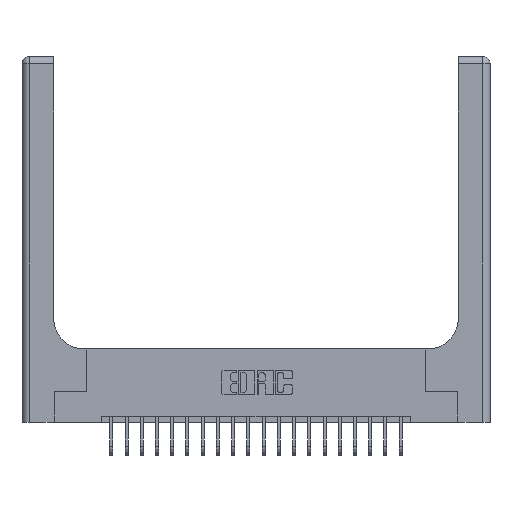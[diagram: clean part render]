
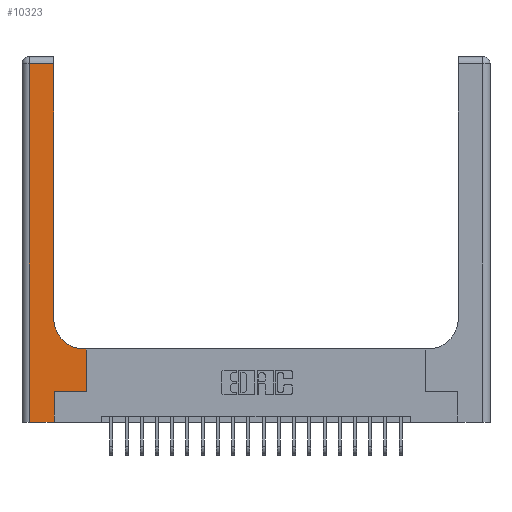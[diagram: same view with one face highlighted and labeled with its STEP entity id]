
A CAD part, top view. The second image highlights one B-rep face of the part: STEP entity #10323.
In plain terms, the highlighted planar face has unit normal (0, 0, 1).
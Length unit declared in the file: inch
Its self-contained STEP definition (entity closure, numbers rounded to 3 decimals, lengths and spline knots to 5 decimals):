
#40 = LINE ( 'NONE', #17816, #15562 ) ;
#163 = CARTESIAN_POINT ( 'NONE',  ( 0., 0., 0.37 ) ) ;
#220 = LINE ( 'NONE', #3405, #14856 ) ;
#269 = DIRECTION ( 'NONE',  ( 1., 0., 0. ) ) ;
#951 = VECTOR ( 'NONE', #11304, 39.37008 ) ;
#1153 = VECTOR ( 'NONE', #1521, 39.37008 ) ;
#1199 = FACE_OUTER_BOUND ( 'NONE', #8722, .T. ) ;
#1295 = EDGE_CURVE ( 'NONE', #9481, #20837, #11228, .T. ) ;
#1521 = DIRECTION ( 'NONE',  ( 0., 1., 0. ) ) ;
#1726 = VECTOR ( 'NONE', #14231, 39.37008 ) ;
#2073 = ORIENTED_EDGE ( 'NONE', *, *, #12295, .T. ) ;
#2400 = VECTOR ( 'NONE', #5917, 39.37008 ) ;
#2632 = CARTESIAN_POINT ( 'NONE',  ( 0.528, 0.6, 0.37 ) ) ;
#2777 = CARTESIAN_POINT ( 'NONE',  ( 0.265, 0.25, 0.37 ) ) ;
#2857 = EDGE_CURVE ( 'NONE', #16329, #14969, #40, .T. ) ;
#2881 = EDGE_CURVE ( 'NONE', #20624, #17365, #4722, .T. ) ;
#3127 = LINE ( 'NONE', #13117, #13596 ) ;
#3227 = CARTESIAN_POINT ( 'NONE',  ( 0.528, 0.25, 0.37 ) ) ;
#3405 = CARTESIAN_POINT ( 'NONE',  ( 0.26, 3., 0.37 ) ) ;
#3665 = VECTOR ( 'NONE', #269, 39.37008 ) ;
#3971 = CARTESIAN_POINT ( 'NONE',  ( 0.26, 2.94, 0.37 ) ) ;
#4101 = EDGE_CURVE ( 'NONE', #17184, #4433, #3127, .T. ) ;
#4433 = VERTEX_POINT ( 'NONE', #15448 ) ;
#4706 = DIRECTION ( 'NONE',  ( 0., 0., -1. ) ) ;
#4722 = LINE ( 'NONE', #11517, #951 ) ;
#5135 = DIRECTION ( 'NONE',  ( 1., 0., 0. ) ) ;
#5807 = CIRCLE ( 'NONE', #8211, 0.25 ) ;
#5917 = DIRECTION ( 'NONE',  ( 0., -1., 0. ) ) ;
#6009 = EDGE_CURVE ( 'NONE', #13041, #16329, #220, .T. ) ;
#6696 = DIRECTION ( 'NONE',  ( 0., 1., 0. ) ) ;
#7517 = LINE ( 'NONE', #18830, #2400 ) ;
#7684 = DIRECTION ( 'NONE',  ( -1., 0., 0. ) ) ;
#7858 = ORIENTED_EDGE ( 'NONE', *, *, #18553, .T. ) ;
#8211 = AXIS2_PLACEMENT_3D ( 'NONE', #13232, #19739, #5135 ) ;
#8507 = ORIENTED_EDGE ( 'NONE', *, *, #1295, .T. ) ;
#8722 = EDGE_LOOP ( 'NONE', ( #18386, #10126, #13275, #8507, #15088, #10303, #7858, #10452, #2073 ) ) ;
#9481 = VERTEX_POINT ( 'NONE', #11335 ) ;
#9556 = EDGE_CURVE ( 'NONE', #20837, #20624, #16253, .T. ) ;
#9654 = CARTESIAN_POINT ( 'NONE',  ( 0.265, 0., 0.37 ) ) ;
#10126 = ORIENTED_EDGE ( 'NONE', *, *, #2857, .T. ) ;
#10303 = ORIENTED_EDGE ( 'NONE', *, *, #2881, .T. ) ;
#10323 = ADVANCED_FACE ( 'NONE', ( #1199 ), #11092, .F. ) ;
#10452 = ORIENTED_EDGE ( 'NONE', *, *, #4101, .T. ) ;
#11092 = PLANE ( 'NONE',  #17394 ) ;
#11228 = LINE ( 'NONE', #163, #3665 ) ;
#11288 = CARTESIAN_POINT ( 'NONE',  ( 0., 3., 0.37 ) ) ;
#11304 = DIRECTION ( 'NONE',  ( 1., 0., 0. ) ) ;
#11335 = CARTESIAN_POINT ( 'NONE',  ( 0.06, 0., 0.37 ) ) ;
#11517 = CARTESIAN_POINT ( 'NONE',  ( 0.265, 0.25, 0.37 ) ) ;
#11621 = EDGE_CURVE ( 'NONE', #14969, #9481, #7517, .T. ) ;
#12295 = EDGE_CURVE ( 'NONE', #4433, #13041, #5807, .T. ) ;
#13041 = VERTEX_POINT ( 'NONE', #20893 ) ;
#13117 = CARTESIAN_POINT ( 'NONE',  ( 0.26, 0.6, 0.37 ) ) ;
#13232 = CARTESIAN_POINT ( 'NONE',  ( 0.51, 0.85, 0.37 ) ) ;
#13275 = ORIENTED_EDGE ( 'NONE', *, *, #11621, .T. ) ;
#13596 = VECTOR ( 'NONE', #20933, 39.37008 ) ;
#14231 = DIRECTION ( 'NONE',  ( 0., 1., 0. ) ) ;
#14856 = VECTOR ( 'NONE', #6696, 39.37008 ) ;
#14969 = VERTEX_POINT ( 'NONE', #17428 ) ;
#15088 = ORIENTED_EDGE ( 'NONE', *, *, #9556, .T. ) ;
#15448 = CARTESIAN_POINT ( 'NONE',  ( 0.51, 0.6, 0.37 ) ) ;
#15562 = VECTOR ( 'NONE', #16113, 39.37008 ) ;
#15916 = CARTESIAN_POINT ( 'NONE',  ( 0.528, 0.25, 0.37 ) ) ;
#16104 = LINE ( 'NONE', #3227, #1153 ) ;
#16113 = DIRECTION ( 'NONE',  ( -1., 0., 0. ) ) ;
#16253 = LINE ( 'NONE', #9654, #1726 ) ;
#16329 = VERTEX_POINT ( 'NONE', #3971 ) ;
#17184 = VERTEX_POINT ( 'NONE', #2632 ) ;
#17365 = VERTEX_POINT ( 'NONE', #15916 ) ;
#17394 = AXIS2_PLACEMENT_3D ( 'NONE', #11288, #4706, #7684 ) ;
#17428 = CARTESIAN_POINT ( 'NONE',  ( 0.06, 2.94, 0.37 ) ) ;
#17816 = CARTESIAN_POINT ( 'NONE',  ( 0., 2.94, 0.37 ) ) ;
#18386 = ORIENTED_EDGE ( 'NONE', *, *, #6009, .T. ) ;
#18553 = EDGE_CURVE ( 'NONE', #17365, #17184, #16104, .T. ) ;
#18830 = CARTESIAN_POINT ( 'NONE',  ( 0.06, 3., 0.37 ) ) ;
#19714 = CARTESIAN_POINT ( 'NONE',  ( 0.265, 0., 0.37 ) ) ;
#19739 = DIRECTION ( 'NONE',  ( 0., 0., -1. ) ) ;
#20624 = VERTEX_POINT ( 'NONE', #2777 ) ;
#20837 = VERTEX_POINT ( 'NONE', #19714 ) ;
#20893 = CARTESIAN_POINT ( 'NONE',  ( 0.26, 0.85, 0.37 ) ) ;
#20933 = DIRECTION ( 'NONE',  ( -1., 0., 0. ) ) ;
